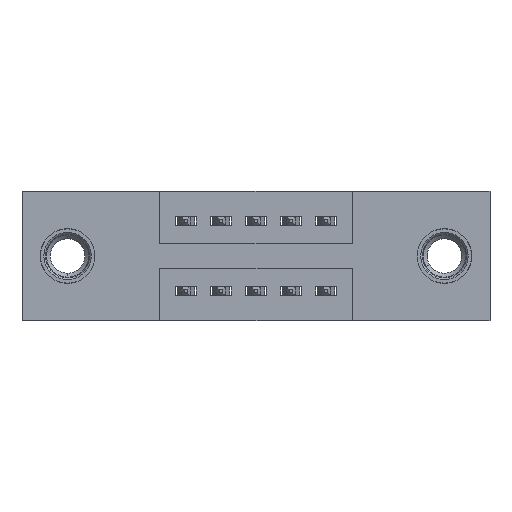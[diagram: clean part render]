
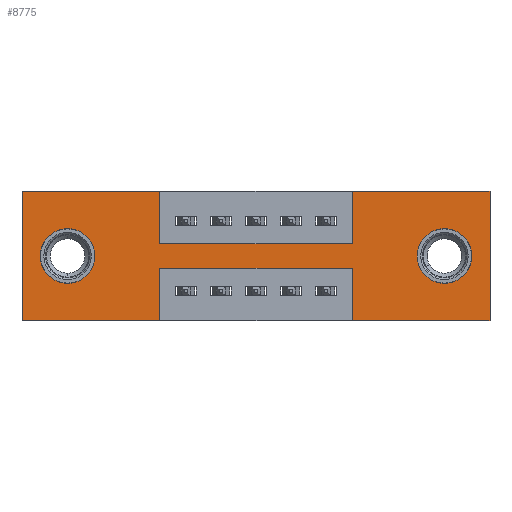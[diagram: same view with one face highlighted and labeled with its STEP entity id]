
A CAD part, front view. The second image highlights one B-rep face of the part: STEP entity #8775.
In plain terms, the highlighted planar face has unit normal (0, -1, 0).
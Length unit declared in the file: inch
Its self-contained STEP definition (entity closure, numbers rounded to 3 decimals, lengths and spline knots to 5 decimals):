
#37 = EDGE_CURVE ( 'NONE', #5459, #9623, #7955, .T. ) ;
#63 = VECTOR ( 'NONE', #3181, 39.37008 ) ;
#141 = LINE ( 'NONE', #4166, #7920 ) ;
#183 = VECTOR ( 'NONE', #8412, 39.37008 ) ;
#312 = ORIENTED_EDGE ( 'NONE', *, *, #37, .F. ) ;
#469 = EDGE_CURVE ( 'NONE', #9623, #2292, #6975, .T. ) ;
#512 = EDGE_CURVE ( 'NONE', #7830, #5459, #808, .T. ) ;
#514 = CARTESIAN_POINT ( 'NONE',  ( 1.205, 0., -0.263 ) ) ;
#573 = DIRECTION ( 'NONE',  ( 1., 0., 0. ) ) ;
#676 = EDGE_CURVE ( 'NONE', #9457, #9467, #1532, .T. ) ;
#718 = EDGE_LOOP ( 'NONE', ( #7666, #1084, #9274, #2885, #4412, #5986, #312, #9751, #3351, #5204, #2147, #7481 ) ) ;
#765 = CARTESIAN_POINT ( 'NONE',  ( 0., 0., 0. ) ) ;
#791 = DIRECTION ( 'NONE',  ( 0., 1., 0. ) ) ;
#808 = LINE ( 'NONE', #9837, #6852 ) ;
#881 = ORIENTED_EDGE ( 'NONE', *, *, #5402, .T. ) ;
#892 = CARTESIAN_POINT ( 'NONE',  ( 0., 0., 0. ) ) ;
#996 = CARTESIAN_POINT ( 'NONE',  ( 0.3925, 0., -0.37 ) ) ;
#1036 = CARTESIAN_POINT ( 'NONE',  ( 0.13, 0., -0.185 ) ) ;
#1084 = ORIENTED_EDGE ( 'NONE', *, *, #8250, .F. ) ;
#1105 = VECTOR ( 'NONE', #4798, 39.37008 ) ;
#1108 = EDGE_CURVE ( 'NONE', #2072, #5050, #2921, .T. ) ;
#1206 = CARTESIAN_POINT ( 'NONE',  ( 0., 0., -0.37 ) ) ;
#1479 = AXIS2_PLACEMENT_3D ( 'NONE', #6317, #8679, #5436 ) ;
#1532 = CIRCLE ( 'NONE', #5271, 0.078 ) ;
#1745 = CARTESIAN_POINT ( 'NONE',  ( 1.205, 0., -0.107 ) ) ;
#1862 = CARTESIAN_POINT ( 'NONE',  ( 0.9425, 0., -0.37 ) ) ;
#1913 = EDGE_CURVE ( 'NONE', #4347, #8209, #3044, .T. ) ;
#1925 = EDGE_CURVE ( 'NONE', #2292, #8378, #2430, .T. ) ;
#1927 = AXIS2_PLACEMENT_3D ( 'NONE', #1206, #7382, #5093 ) ;
#2011 = VERTEX_POINT ( 'NONE', #5709 ) ;
#2072 = VERTEX_POINT ( 'NONE', #1862 ) ;
#2077 = DIRECTION ( 'NONE',  ( 0., 0., 1. ) ) ;
#2147 = ORIENTED_EDGE ( 'NONE', *, *, #8638, .F. ) ;
#2213 = LINE ( 'NONE', #4230, #3923 ) ;
#2292 = VERTEX_POINT ( 'NONE', #5878 ) ;
#2302 = CARTESIAN_POINT ( 'NONE',  ( 1.335, 0., -0.37 ) ) ;
#2325 = VECTOR ( 'NONE', #4206, 39.37008 ) ;
#2336 = VECTOR ( 'NONE', #573, 39.37008 ) ;
#2430 = LINE ( 'NONE', #2570, #5524 ) ;
#2434 = DIRECTION ( 'NONE',  ( 1., 0., 0. ) ) ;
#2570 = CARTESIAN_POINT ( 'NONE',  ( 1.335, 0., 0. ) ) ;
#2885 = ORIENTED_EDGE ( 'NONE', *, *, #4969, .F. ) ;
#2921 = LINE ( 'NONE', #6195, #183 ) ;
#3044 = LINE ( 'NONE', #892, #9060 ) ;
#3181 = DIRECTION ( 'NONE',  ( 0., 0., 1. ) ) ;
#3206 = AXIS2_PLACEMENT_3D ( 'NONE', #6251, #791, #8566 ) ;
#3286 = FACE_BOUND ( 'NONE', #6637, .T. ) ;
#3304 = DIRECTION ( 'NONE',  ( 0., 0., -1. ) ) ;
#3351 = ORIENTED_EDGE ( 'NONE', *, *, #9716, .F. ) ;
#3383 = VERTEX_POINT ( 'NONE', #1745 ) ;
#3716 = LINE ( 'NONE', #4901, #1105 ) ;
#3775 = CARTESIAN_POINT ( 'NONE',  ( 0.3925, 0., 0. ) ) ;
#3923 = VECTOR ( 'NONE', #3304, 39.37008 ) ;
#4009 = DIRECTION ( 'NONE',  ( 0., 1., 0. ) ) ;
#4075 = EDGE_CURVE ( 'NONE', #9467, #9457, #8286, .T. ) ;
#4166 = CARTESIAN_POINT ( 'NONE',  ( 0.3925, 0., 0. ) ) ;
#4206 = DIRECTION ( 'NONE',  ( 0., 0., 1. ) ) ;
#4230 = CARTESIAN_POINT ( 'NONE',  ( 0.3925, 0., -0.37 ) ) ;
#4347 = VERTEX_POINT ( 'NONE', #6696 ) ;
#4412 = ORIENTED_EDGE ( 'NONE', *, *, #1925, .F. ) ;
#4487 = EDGE_CURVE ( 'NONE', #6323, #2011, #8270, .T. ) ;
#4798 = DIRECTION ( 'NONE',  ( -1., 0., 0. ) ) ;
#4901 = CARTESIAN_POINT ( 'NONE',  ( 0., 0., -0.37 ) ) ;
#4908 = ORIENTED_EDGE ( 'NONE', *, *, #4075, .T. ) ;
#4936 = DIRECTION ( 'NONE',  ( 0., 0., -1. ) ) ;
#4969 = EDGE_CURVE ( 'NONE', #8378, #2072, #3716, .T. ) ;
#5050 = VERTEX_POINT ( 'NONE', #9758 ) ;
#5093 = DIRECTION ( 'NONE',  ( 0., 0., -1. ) ) ;
#5204 = ORIENTED_EDGE ( 'NONE', *, *, #1913, .F. ) ;
#5271 = AXIS2_PLACEMENT_3D ( 'NONE', #1036, #8087, #2077 ) ;
#5402 = EDGE_CURVE ( 'NONE', #7529, #3383, #5834, .T. ) ;
#5436 = DIRECTION ( 'NONE',  ( 0., 0., -1. ) ) ;
#5459 = VERTEX_POINT ( 'NONE', #9300 ) ;
#5524 = VECTOR ( 'NONE', #9374, 39.37008 ) ;
#5671 = DIRECTION ( 'NONE',  ( 0., 0., 1. ) ) ;
#5709 = CARTESIAN_POINT ( 'NONE',  ( 0., 0., -0.37 ) ) ;
#5834 = CIRCLE ( 'NONE', #3206, 0.078 ) ;
#5878 = CARTESIAN_POINT ( 'NONE',  ( 1.335, 0., 0. ) ) ;
#5902 = LINE ( 'NONE', #765, #63 ) ;
#5908 = LINE ( 'NONE', #6810, #9064 ) ;
#5986 = ORIENTED_EDGE ( 'NONE', *, *, #469, .F. ) ;
#6056 = DIRECTION ( 'NONE',  ( 1., 0., 0. ) ) ;
#6074 = DIRECTION ( 'NONE',  ( -1., 0., 0. ) ) ;
#6146 = DIRECTION ( 'NONE',  ( -1., 0., 0. ) ) ;
#6160 = ORIENTED_EDGE ( 'NONE', *, *, #676, .T. ) ;
#6195 = CARTESIAN_POINT ( 'NONE',  ( 0.9425, 0., -0.37 ) ) ;
#6225 = CARTESIAN_POINT ( 'NONE',  ( 0.3925, 0., -0.22 ) ) ;
#6251 = CARTESIAN_POINT ( 'NONE',  ( 1.205, 0., -0.185 ) ) ;
#6317 = CARTESIAN_POINT ( 'NONE',  ( 1.205, 0., -0.185 ) ) ;
#6323 = VERTEX_POINT ( 'NONE', #996 ) ;
#6527 = CARTESIAN_POINT ( 'NONE',  ( 0.9425, 0., 0. ) ) ;
#6564 = PLANE ( 'NONE',  #1927 ) ;
#6637 = EDGE_LOOP ( 'NONE', ( #6160, #4908 ) ) ;
#6678 = EDGE_CURVE ( 'NONE', #3383, #7529, #9672, .T. ) ;
#6696 = CARTESIAN_POINT ( 'NONE',  ( 0., 0., 0. ) ) ;
#6810 = CARTESIAN_POINT ( 'NONE',  ( 0.3925, 0., -0.22 ) ) ;
#6852 = VECTOR ( 'NONE', #2434, 39.37008 ) ;
#6909 = CARTESIAN_POINT ( 'NONE',  ( 0.13, 0., -0.107 ) ) ;
#6975 = LINE ( 'NONE', #9120, #2336 ) ;
#6981 = CARTESIAN_POINT ( 'NONE',  ( 0., 0., -0.37 ) ) ;
#7320 = EDGE_LOOP ( 'NONE', ( #7913, #881 ) ) ;
#7382 = DIRECTION ( 'NONE',  ( 0., -1., 0. ) ) ;
#7481 = ORIENTED_EDGE ( 'NONE', *, *, #4487, .F. ) ;
#7505 = VECTOR ( 'NONE', #6146, 39.37008 ) ;
#7529 = VERTEX_POINT ( 'NONE', #514 ) ;
#7666 = ORIENTED_EDGE ( 'NONE', *, *, #7982, .F. ) ;
#7731 = VERTEX_POINT ( 'NONE', #6225 ) ;
#7813 = CARTESIAN_POINT ( 'NONE',  ( 0.3925, 0., -0.15 ) ) ;
#7830 = VERTEX_POINT ( 'NONE', #7813 ) ;
#7913 = ORIENTED_EDGE ( 'NONE', *, *, #6678, .T. ) ;
#7920 = VECTOR ( 'NONE', #4936, 39.37008 ) ;
#7955 = LINE ( 'NONE', #6527, #2325 ) ;
#7982 = EDGE_CURVE ( 'NONE', #7731, #6323, #2213, .T. ) ;
#8087 = DIRECTION ( 'NONE',  ( 0., 1., 0. ) ) ;
#8209 = VERTEX_POINT ( 'NONE', #3775 ) ;
#8250 = EDGE_CURVE ( 'NONE', #5050, #7731, #5908, .T. ) ;
#8270 = LINE ( 'NONE', #6981, #7505 ) ;
#8286 = CIRCLE ( 'NONE', #9030, 0.078 ) ;
#8378 = VERTEX_POINT ( 'NONE', #2302 ) ;
#8412 = DIRECTION ( 'NONE',  ( 0., 0., 1. ) ) ;
#8566 = DIRECTION ( 'NONE',  ( 0., 0., -1. ) ) ;
#8638 = EDGE_CURVE ( 'NONE', #2011, #4347, #5902, .T. ) ;
#8679 = DIRECTION ( 'NONE',  ( 0., 1., 0. ) ) ;
#8688 = FACE_OUTER_BOUND ( 'NONE', #718, .T. ) ;
#8693 = CARTESIAN_POINT ( 'NONE',  ( 0.13, 0., -0.185 ) ) ;
#8775 = ADVANCED_FACE ( 'NONE', ( #10063, #3286, #8688 ), #6564, .T. ) ;
#9030 = AXIS2_PLACEMENT_3D ( 'NONE', #8693, #4009, #5671 ) ;
#9060 = VECTOR ( 'NONE', #6056, 39.37008 ) ;
#9064 = VECTOR ( 'NONE', #6074, 39.37008 ) ;
#9120 = CARTESIAN_POINT ( 'NONE',  ( 0., 0., 0. ) ) ;
#9274 = ORIENTED_EDGE ( 'NONE', *, *, #1108, .F. ) ;
#9300 = CARTESIAN_POINT ( 'NONE',  ( 0.9425, 0., -0.15 ) ) ;
#9303 = CARTESIAN_POINT ( 'NONE',  ( 0.13, 0., -0.263 ) ) ;
#9374 = DIRECTION ( 'NONE',  ( 0., 0., -1. ) ) ;
#9457 = VERTEX_POINT ( 'NONE', #6909 ) ;
#9467 = VERTEX_POINT ( 'NONE', #9303 ) ;
#9515 = CARTESIAN_POINT ( 'NONE',  ( 0.9425, 0., 0. ) ) ;
#9623 = VERTEX_POINT ( 'NONE', #9515 ) ;
#9672 = CIRCLE ( 'NONE', #1479, 0.078 ) ;
#9716 = EDGE_CURVE ( 'NONE', #8209, #7830, #141, .T. ) ;
#9751 = ORIENTED_EDGE ( 'NONE', *, *, #512, .F. ) ;
#9758 = CARTESIAN_POINT ( 'NONE',  ( 0.9425, 0., -0.22 ) ) ;
#9837 = CARTESIAN_POINT ( 'NONE',  ( 0.3925, 0., -0.15 ) ) ;
#10063 = FACE_BOUND ( 'NONE', #7320, .T. ) ;
